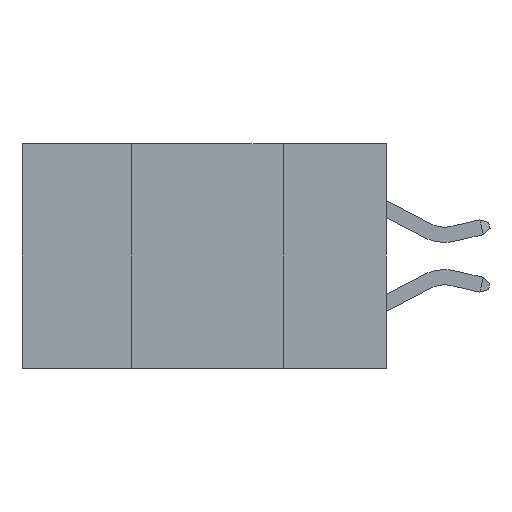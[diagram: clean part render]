
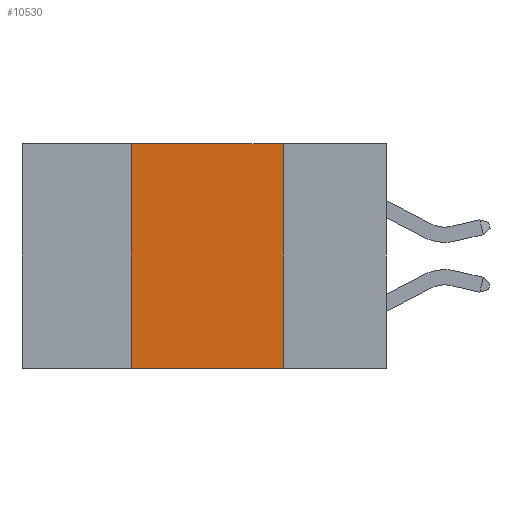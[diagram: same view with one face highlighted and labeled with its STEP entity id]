
A CAD part, left-side view. The second image highlights one B-rep face of the part: STEP entity #10530.
In plain terms, the highlighted planar face has unit normal (-1, 0, 0).
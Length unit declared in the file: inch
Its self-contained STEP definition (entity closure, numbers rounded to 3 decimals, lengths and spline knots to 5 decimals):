
#3000 = VECTOR ( 'NONE', #25868, 39.37008 ) ;
#3065 = AXIS2_PLACEMENT_3D ( 'NONE', #28150, #12625, #8205 ) ;
#3444 = CARTESIAN_POINT ( 'NONE',  ( 0., 0.6, -0.37 ) ) ;
#3619 = CARTESIAN_POINT ( 'NONE',  ( 0., 0.17, -0.37 ) ) ;
#3706 = PLANE ( 'NONE',  #3065 ) ;
#4178 = LINE ( 'NONE', #3444, #27180 ) ;
#5797 = CARTESIAN_POINT ( 'NONE',  ( 0., 0.17, 0. ) ) ;
#6512 = VERTEX_POINT ( 'NONE', #5797 ) ;
#6981 = VECTOR ( 'NONE', #23464, 39.37008 ) ;
#7217 = CARTESIAN_POINT ( 'NONE',  ( 0., 0.42, 0. ) ) ;
#7885 = CARTESIAN_POINT ( 'NONE',  ( 0., 0.6, 0. ) ) ;
#8205 = DIRECTION ( 'NONE',  ( 0., 0., -1. ) ) ;
#9446 = DIRECTION ( 'NONE',  ( 0., 0., 1. ) ) ;
#9604 = LINE ( 'NONE', #7217, #25258 ) ;
#9617 = VERTEX_POINT ( 'NONE', #15758 ) ;
#10300 = CARTESIAN_POINT ( 'NONE',  ( 0., 0.17, 0. ) ) ;
#10530 = ADVANCED_FACE ( 'NONE', ( #21029 ), #3706, .F. ) ;
#11329 = ORIENTED_EDGE ( 'NONE', *, *, #17799, .F. ) ;
#12040 = CARTESIAN_POINT ( 'NONE',  ( 0., 0.42, -0.37 ) ) ;
#12070 = EDGE_CURVE ( 'NONE', #16693, #12757, #4178, .T. ) ;
#12625 = DIRECTION ( 'NONE',  ( 1., 0., 0. ) ) ;
#12757 = VERTEX_POINT ( 'NONE', #3619 ) ;
#14107 = ORIENTED_EDGE ( 'NONE', *, *, #19350, .F. ) ;
#15758 = CARTESIAN_POINT ( 'NONE',  ( 0., 0.42, 0. ) ) ;
#16693 = VERTEX_POINT ( 'NONE', #12040 ) ;
#17243 = ORIENTED_EDGE ( 'NONE', *, *, #12070, .T. ) ;
#17425 = LINE ( 'NONE', #7885, #6981 ) ;
#17799 = EDGE_CURVE ( 'NONE', #16693, #9617, #9604, .T. ) ;
#19350 = EDGE_CURVE ( 'NONE', #9617, #6512, #17425, .T. ) ;
#19938 = ORIENTED_EDGE ( 'NONE', *, *, #27885, .F. ) ;
#20168 = LINE ( 'NONE', #10300, #3000 ) ;
#21029 = FACE_OUTER_BOUND ( 'NONE', #22255, .T. ) ;
#21338 = DIRECTION ( 'NONE',  ( 0., -1., 0. ) ) ;
#22255 = EDGE_LOOP ( 'NONE', ( #19938, #14107, #11329, #17243 ) ) ;
#23464 = DIRECTION ( 'NONE',  ( 0., -1., 0. ) ) ;
#25258 = VECTOR ( 'NONE', #9446, 39.37008 ) ;
#25868 = DIRECTION ( 'NONE',  ( 0., 0., -1. ) ) ;
#27180 = VECTOR ( 'NONE', #21338, 39.37008 ) ;
#27885 = EDGE_CURVE ( 'NONE', #6512, #12757, #20168, .T. ) ;
#28150 = CARTESIAN_POINT ( 'NONE',  ( 0., 0.6, 0. ) ) ;
